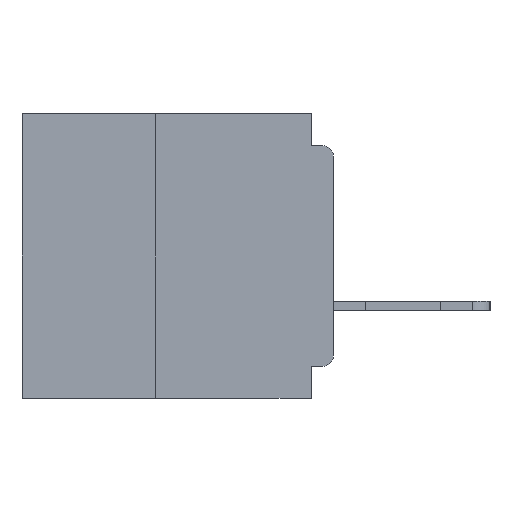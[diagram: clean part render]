
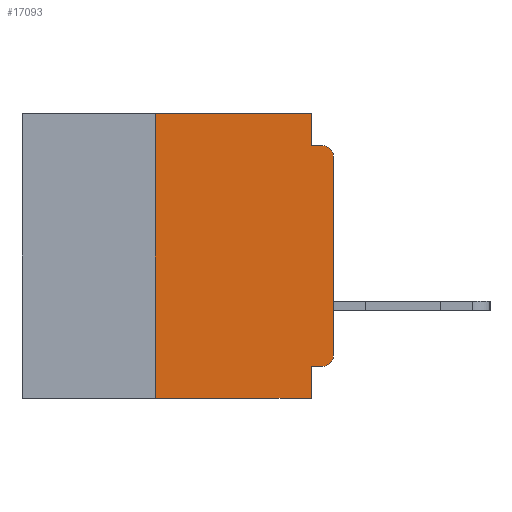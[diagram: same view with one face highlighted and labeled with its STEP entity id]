
A CAD part, left-side view. The second image highlights one B-rep face of the part: STEP entity #17093.
In plain terms, the highlighted planar face has unit normal (-1, 0, 0).
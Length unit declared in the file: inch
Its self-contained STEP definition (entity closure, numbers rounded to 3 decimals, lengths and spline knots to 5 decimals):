
#159 = ORIENTED_EDGE ( 'NONE', *, *, #7243, .T. ) ;
#889 = CIRCLE ( 'NONE', #9027, 0.015 ) ;
#1110 = CARTESIAN_POINT ( 'NONE',  ( 0., 0.437, -0.4 ) ) ;
#1211 = EDGE_CURVE ( 'NONE', #7136, #9226, #37389, .T. ) ;
#1717 = FACE_OUTER_BOUND ( 'NONE', #37313, .T. ) ;
#2922 = CARTESIAN_POINT ( 'NONE',  ( 0., 0., -0.045 ) ) ;
#3011 = DIRECTION ( 'NONE',  ( 0., -1., 0. ) ) ;
#3193 = LINE ( 'NONE', #26061, #33473 ) ;
#3327 = EDGE_CURVE ( 'NONE', #19277, #9779, #889, .T. ) ;
#3632 = DIRECTION ( 'NONE',  ( 0., 0., 1. ) ) ;
#3714 = ORIENTED_EDGE ( 'NONE', *, *, #1211, .F. ) ;
#4011 = CARTESIAN_POINT ( 'NONE',  ( 0., 0.015, -0.045 ) ) ;
#4102 = LINE ( 'NONE', #18230, #35321 ) ;
#4189 = CARTESIAN_POINT ( 'NONE',  ( 0., 0.015, -0.34 ) ) ;
#4832 = VERTEX_POINT ( 'NONE', #12989 ) ;
#5085 = CARTESIAN_POINT ( 'NONE',  ( 0., 0.031, -0.4 ) ) ;
#6381 = VECTOR ( 'NONE', #26407, 39.37008 ) ;
#6399 = ORIENTED_EDGE ( 'NONE', *, *, #11188, .F. ) ;
#6541 = PLANE ( 'NONE',  #15103 ) ;
#6742 = VERTEX_POINT ( 'NONE', #27446 ) ;
#6910 = DIRECTION ( 'NONE',  ( 0., 0., -1. ) ) ;
#6939 = EDGE_CURVE ( 'NONE', #4832, #30935, #3193, .T. ) ;
#6956 = DIRECTION ( 'NONE',  ( -1., 0., 0. ) ) ;
#7001 = CARTESIAN_POINT ( 'NONE',  ( 0., 0.015, -0.06 ) ) ;
#7136 = VERTEX_POINT ( 'NONE', #32828 ) ;
#7189 = DIRECTION ( 'NONE',  ( 0., 0., -1. ) ) ;
#7243 = EDGE_CURVE ( 'NONE', #7136, #6742, #32076, .T. ) ;
#7317 = LINE ( 'NONE', #2922, #6381 ) ;
#7437 = LINE ( 'NONE', #10861, #15168 ) ;
#8056 = CARTESIAN_POINT ( 'NONE',  ( 0., 0.031, 0. ) ) ;
#9027 = AXIS2_PLACEMENT_3D ( 'NONE', #7001, #6956, #6910 ) ;
#9226 = VERTEX_POINT ( 'NONE', #22282 ) ;
#9779 = VERTEX_POINT ( 'NONE', #4011 ) ;
#9891 = DIRECTION ( 'NONE',  ( 0., -1., 0. ) ) ;
#9972 = ORIENTED_EDGE ( 'NONE', *, *, #13388, .T. ) ;
#10861 = CARTESIAN_POINT ( 'NONE',  ( 0., 0.031, 0. ) ) ;
#11188 = EDGE_CURVE ( 'NONE', #30935, #6742, #17074, .T. ) ;
#11342 = EDGE_CURVE ( 'NONE', #9226, #13057, #35878, .T. ) ;
#12394 = DIRECTION ( 'NONE',  ( 0., 0., -1. ) ) ;
#12989 = CARTESIAN_POINT ( 'NONE',  ( 0., 0.015, -0.355 ) ) ;
#13057 = VERTEX_POINT ( 'NONE', #8056 ) ;
#13388 = EDGE_CURVE ( 'NONE', #20194, #19277, #4102, .T. ) ;
#13904 = DIRECTION ( 'NONE',  ( 0., 0., -1. ) ) ;
#15103 = AXIS2_PLACEMENT_3D ( 'NONE', #29834, #29963, #12394 ) ;
#15168 = VECTOR ( 'NONE', #22649, 39.37008 ) ;
#16923 = EDGE_CURVE ( 'NONE', #24504, #9779, #7317, .T. ) ;
#17074 = LINE ( 'NONE', #5085, #23967 ) ;
#17093 = ADVANCED_FACE ( 'NONE', ( #1717 ), #6541, .F. ) ;
#17657 = CARTESIAN_POINT ( 'NONE',  ( 0., 0.031, -0.045 ) ) ;
#17886 = ORIENTED_EDGE ( 'NONE', *, *, #16923, .F. ) ;
#18230 = CARTESIAN_POINT ( 'NONE',  ( 0., 0., 0. ) ) ;
#18310 = AXIS2_PLACEMENT_3D ( 'NONE', #4189, #24724, #7189 ) ;
#19277 = VERTEX_POINT ( 'NONE', #28657 ) ;
#20194 = VERTEX_POINT ( 'NONE', #33083 ) ;
#20549 = CARTESIAN_POINT ( 'NONE',  ( 0., 0.437, 0. ) ) ;
#21754 = VECTOR ( 'NONE', #23978, 39.37008 ) ;
#21776 = CIRCLE ( 'NONE', #18310, 0.015 ) ;
#22282 = CARTESIAN_POINT ( 'NONE',  ( 0., 0.25, 0. ) ) ;
#22649 = DIRECTION ( 'NONE',  ( 0., 0., -1. ) ) ;
#23967 = VECTOR ( 'NONE', #13904, 39.37008 ) ;
#23978 = DIRECTION ( 'NONE',  ( 0., 0., 1. ) ) ;
#24504 = VERTEX_POINT ( 'NONE', #17657 ) ;
#24724 = DIRECTION ( 'NONE',  ( -1., 0., 0. ) ) ;
#25223 = VECTOR ( 'NONE', #9891, 39.37008 ) ;
#26061 = CARTESIAN_POINT ( 'NONE',  ( 0., 0., -0.355 ) ) ;
#26407 = DIRECTION ( 'NONE',  ( 0., -1., 0. ) ) ;
#27388 = CARTESIAN_POINT ( 'NONE',  ( 0., 0.031, -0.355 ) ) ;
#27446 = CARTESIAN_POINT ( 'NONE',  ( 0., 0.031, -0.4 ) ) ;
#27460 = EDGE_CURVE ( 'NONE', #13057, #24504, #7437, .T. ) ;
#28657 = CARTESIAN_POINT ( 'NONE',  ( 0., 0., -0.06 ) ) ;
#29699 = ORIENTED_EDGE ( 'NONE', *, *, #3327, .T. ) ;
#29834 = CARTESIAN_POINT ( 'NONE',  ( 0., 0.437, 0. ) ) ;
#29963 = DIRECTION ( 'NONE',  ( 1., 0., 0. ) ) ;
#30935 = VERTEX_POINT ( 'NONE', #27388 ) ;
#30966 = EDGE_CURVE ( 'NONE', #4832, #20194, #21776, .T. ) ;
#31359 = ORIENTED_EDGE ( 'NONE', *, *, #11342, .F. ) ;
#32076 = LINE ( 'NONE', #1110, #25223 ) ;
#32492 = ORIENTED_EDGE ( 'NONE', *, *, #30966, .T. ) ;
#32828 = CARTESIAN_POINT ( 'NONE',  ( 0., 0.25, -0.4 ) ) ;
#33083 = CARTESIAN_POINT ( 'NONE',  ( 0., 0., -0.34 ) ) ;
#33473 = VECTOR ( 'NONE', #34898, 39.37008 ) ;
#34052 = VECTOR ( 'NONE', #3011, 39.37008 ) ;
#34898 = DIRECTION ( 'NONE',  ( 0., 1., 0. ) ) ;
#35058 = ORIENTED_EDGE ( 'NONE', *, *, #27460, .F. ) ;
#35234 = CARTESIAN_POINT ( 'NONE',  ( 0., 0.25, -0.4 ) ) ;
#35321 = VECTOR ( 'NONE', #3632, 39.37008 ) ;
#35322 = ORIENTED_EDGE ( 'NONE', *, *, #6939, .F. ) ;
#35878 = LINE ( 'NONE', #20549, #34052 ) ;
#37313 = EDGE_LOOP ( 'NONE', ( #9972, #29699, #17886, #35058, #31359, #3714, #159, #6399, #35322, #32492 ) ) ;
#37389 = LINE ( 'NONE', #35234, #21754 ) ;
